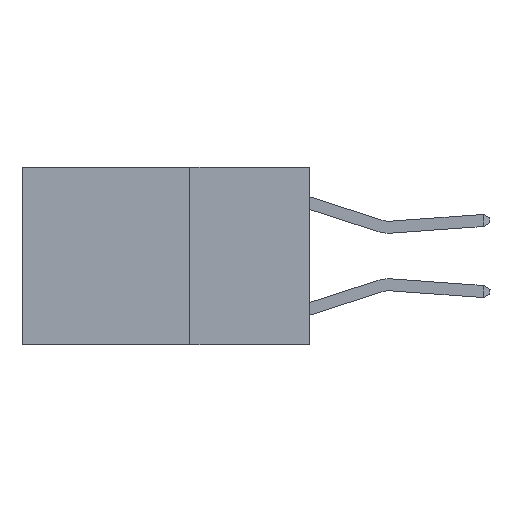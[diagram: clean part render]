
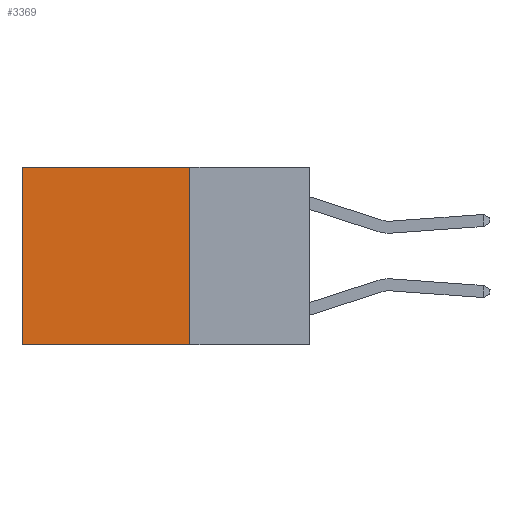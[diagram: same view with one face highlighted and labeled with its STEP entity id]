
A CAD part, left-side view. The second image highlights one B-rep face of the part: STEP entity #3369.
In plain terms, the highlighted planar face has unit normal (-1, 0, 0).
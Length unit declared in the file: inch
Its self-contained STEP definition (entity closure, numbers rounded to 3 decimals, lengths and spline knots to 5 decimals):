
#109 = EDGE_CURVE ( 'NONE', #11187, #10267, #3211, .T. ) ;
#532 = CARTESIAN_POINT ( 'NONE',  ( 0.2625, 0.25, -0.37 ) ) ;
#1036 = DIRECTION ( 'NONE',  ( 0., 0., -1. ) ) ;
#1185 = VERTEX_POINT ( 'NONE', #5999 ) ;
#1510 = EDGE_CURVE ( 'NONE', #9164, #11187, #9835, .T. ) ;
#1920 = EDGE_CURVE ( 'NONE', #9164, #1185, #14678, .T. ) ;
#2130 = EDGE_CURVE ( 'NONE', #1185, #10267, #7523, .T. ) ;
#2288 = CARTESIAN_POINT ( 'NONE',  ( 0.2625, 0.25, 0. ) ) ;
#2384 = DIRECTION ( 'NONE',  ( 0., 0., -1. ) ) ;
#2563 = FACE_OUTER_BOUND ( 'NONE', #15333, .T. ) ;
#3211 = LINE ( 'NONE', #4851, #10917 ) ;
#3369 = ADVANCED_FACE ( 'NONE', ( #2563 ), #18687, .F. ) ;
#4851 = CARTESIAN_POINT ( 'NONE',  ( 0.2625, 0.25, -0.37 ) ) ;
#5999 = CARTESIAN_POINT ( 'NONE',  ( 0.2625, 0.6, 0. ) ) ;
#6062 = DIRECTION ( 'NONE',  ( 1., 0., 0. ) ) ;
#7523 = LINE ( 'NONE', #13869, #19915 ) ;
#9080 = AXIS2_PLACEMENT_3D ( 'NONE', #18483, #6062, #1036 ) ;
#9164 = VERTEX_POINT ( 'NONE', #2288 ) ;
#9375 = ORIENTED_EDGE ( 'NONE', *, *, #109, .F. ) ;
#9835 = LINE ( 'NONE', #18083, #19547 ) ;
#10267 = VERTEX_POINT ( 'NONE', #20106 ) ;
#10703 = ORIENTED_EDGE ( 'NONE', *, *, #2130, .T. ) ;
#10917 = VECTOR ( 'NONE', #11204, 39.37008 ) ;
#11187 = VERTEX_POINT ( 'NONE', #532 ) ;
#11204 = DIRECTION ( 'NONE',  ( 0., 1., 0. ) ) ;
#13869 = CARTESIAN_POINT ( 'NONE',  ( 0.2625, 0.6, 0. ) ) ;
#14516 = ORIENTED_EDGE ( 'NONE', *, *, #1510, .F. ) ;
#14678 = LINE ( 'NONE', #16403, #18568 ) ;
#15333 = EDGE_LOOP ( 'NONE', ( #10703, #9375, #14516, #15647 ) ) ;
#15647 = ORIENTED_EDGE ( 'NONE', *, *, #1920, .T. ) ;
#16403 = CARTESIAN_POINT ( 'NONE',  ( 0.2625, 0.25, 0. ) ) ;
#18083 = CARTESIAN_POINT ( 'NONE',  ( 0.2625, 0.25, 0. ) ) ;
#18483 = CARTESIAN_POINT ( 'NONE',  ( 0.2625, 0.25, 0. ) ) ;
#18568 = VECTOR ( 'NONE', #19225, 39.37008 ) ;
#18687 = PLANE ( 'NONE',  #9080 ) ;
#19225 = DIRECTION ( 'NONE',  ( 0., 1., 0. ) ) ;
#19547 = VECTOR ( 'NONE', #2384, 39.37008 ) ;
#19915 = VECTOR ( 'NONE', #20152, 39.37008 ) ;
#20106 = CARTESIAN_POINT ( 'NONE',  ( 0.2625, 0.6, -0.37 ) ) ;
#20152 = DIRECTION ( 'NONE',  ( 0., 0., -1. ) ) ;
